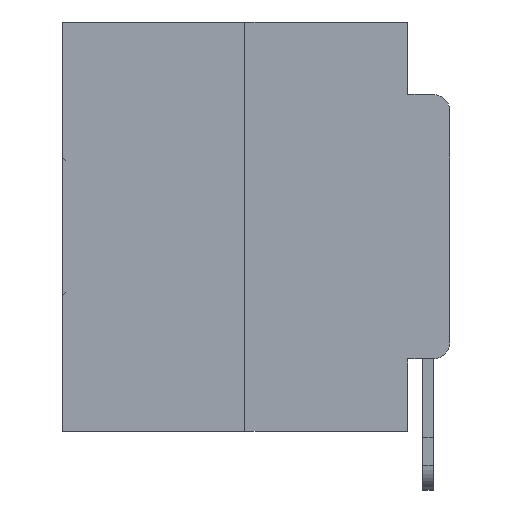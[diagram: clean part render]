
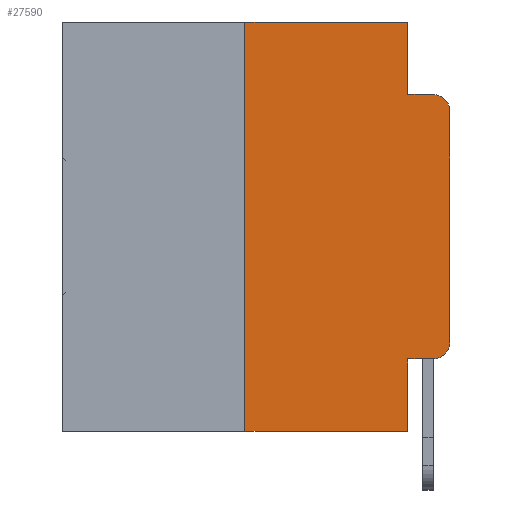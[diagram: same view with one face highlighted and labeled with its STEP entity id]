
A CAD part, left-side view. The second image highlights one B-rep face of the part: STEP entity #27590.
In plain terms, the highlighted planar face has unit normal (-1, 0, 0).
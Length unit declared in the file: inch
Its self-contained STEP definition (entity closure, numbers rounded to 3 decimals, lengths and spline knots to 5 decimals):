
#159 = DIRECTION ( 'NONE',  ( 0., -1., 0. ) ) ;
#421 = EDGE_CURVE ( 'NONE', #21652, #29234, #27852, .T. ) ;
#445 = ORIENTED_EDGE ( 'NONE', *, *, #11988, .T. ) ;
#767 = EDGE_CURVE ( 'NONE', #23382, #13753, #8471, .T. ) ;
#1017 = LINE ( 'NONE', #3094, #6237 ) ;
#1103 = CARTESIAN_POINT ( 'NONE',  ( 0., 0.051, -0.4115 ) ) ;
#1565 = ORIENTED_EDGE ( 'NONE', *, *, #421, .T. ) ;
#3057 = LINE ( 'NONE', #16010, #3883 ) ;
#3094 = CARTESIAN_POINT ( 'NONE',  ( 0., 0.25, 0. ) ) ;
#3330 = CARTESIAN_POINT ( 'NONE',  ( 0., 0.051, 0. ) ) ;
#3883 = VECTOR ( 'NONE', #29842, 39.37008 ) ;
#3971 = CIRCLE ( 'NONE', #16926, 0.02 ) ;
#3992 = ORIENTED_EDGE ( 'NONE', *, *, #29808, .F. ) ;
#4170 = AXIS2_PLACEMENT_3D ( 'NONE', #18735, #4355, #21090 ) ;
#4355 = DIRECTION ( 'NONE',  ( -1., 0., 0. ) ) ;
#5040 = VERTEX_POINT ( 'NONE', #10767 ) ;
#5738 = VERTEX_POINT ( 'NONE', #11638 ) ;
#6237 = VECTOR ( 'NONE', #15291, 39.37008 ) ;
#7415 = LINE ( 'NONE', #14215, #30066 ) ;
#7558 = CARTESIAN_POINT ( 'NONE',  ( 0., 0., 0. ) ) ;
#7598 = CARTESIAN_POINT ( 'NONE',  ( 0., 0.25, 0. ) ) ;
#7911 = PLANE ( 'NONE',  #27528 ) ;
#8407 = DIRECTION ( 'NONE',  ( 0., 0., -1. ) ) ;
#8471 = LINE ( 'NONE', #19296, #27109 ) ;
#8512 = EDGE_CURVE ( 'NONE', #14892, #15529, #7415, .T. ) ;
#9954 = ORIENTED_EDGE ( 'NONE', *, *, #8512, .T. ) ;
#10033 = VERTEX_POINT ( 'NONE', #21681 ) ;
#10429 = DIRECTION ( 'NONE',  ( 0., 0., -1. ) ) ;
#10767 = CARTESIAN_POINT ( 'NONE',  ( 0., 0.051, -0.0885 ) ) ;
#10844 = LINE ( 'NONE', #20130, #21762 ) ;
#11638 = CARTESIAN_POINT ( 'NONE',  ( 0., 0., -0.3915 ) ) ;
#11988 = EDGE_CURVE ( 'NONE', #5738, #10033, #22159, .T. ) ;
#12777 = EDGE_CURVE ( 'NONE', #13753, #5040, #10844, .T. ) ;
#13014 = CARTESIAN_POINT ( 'NONE',  ( 0., 0.02, -0.3915 ) ) ;
#13753 = VERTEX_POINT ( 'NONE', #20800 ) ;
#14215 = CARTESIAN_POINT ( 'NONE',  ( 0., 0.473, -0.5 ) ) ;
#14318 = CARTESIAN_POINT ( 'NONE',  ( 0., 0.051, -0.5 ) ) ;
#14400 = FACE_OUTER_BOUND ( 'NONE', #30806, .T. ) ;
#14892 = VERTEX_POINT ( 'NONE', #26892 ) ;
#15018 = CARTESIAN_POINT ( 'NONE',  ( 0., 0.473, 0. ) ) ;
#15291 = DIRECTION ( 'NONE',  ( 0., 0., 1. ) ) ;
#15359 = DIRECTION ( 'NONE',  ( 0., 0., -1. ) ) ;
#15529 = VERTEX_POINT ( 'NONE', #14318 ) ;
#15917 = CARTESIAN_POINT ( 'NONE',  ( 0., 0.02, -0.4115 ) ) ;
#16010 = CARTESIAN_POINT ( 'NONE',  ( 0., 0.051, -0.0885 ) ) ;
#16163 = ORIENTED_EDGE ( 'NONE', *, *, #767, .F. ) ;
#16926 = AXIS2_PLACEMENT_3D ( 'NONE', #13014, #29201, #15359 ) ;
#18274 = CARTESIAN_POINT ( 'NONE',  ( 0., 0.02, -0.0885 ) ) ;
#18735 = CARTESIAN_POINT ( 'NONE',  ( 0., 0.02, -0.1085 ) ) ;
#19296 = CARTESIAN_POINT ( 'NONE',  ( 0., 0.473, 0. ) ) ;
#19758 = EDGE_CURVE ( 'NONE', #10033, #30638, #20599, .T. ) ;
#20130 = CARTESIAN_POINT ( 'NONE',  ( 0., 0.051, 0. ) ) ;
#20512 = ORIENTED_EDGE ( 'NONE', *, *, #22132, .F. ) ;
#20599 = CIRCLE ( 'NONE', #4170, 0.02 ) ;
#20800 = CARTESIAN_POINT ( 'NONE',  ( 0., 0.051, 0. ) ) ;
#20803 = EDGE_CURVE ( 'NONE', #29234, #5738, #3971, .T. ) ;
#20974 = ORIENTED_EDGE ( 'NONE', *, *, #12777, .F. ) ;
#21006 = VECTOR ( 'NONE', #159, 39.37008 ) ;
#21090 = DIRECTION ( 'NONE',  ( 0., 0., -1. ) ) ;
#21322 = ORIENTED_EDGE ( 'NONE', *, *, #19758, .T. ) ;
#21652 = VERTEX_POINT ( 'NONE', #1103 ) ;
#21681 = CARTESIAN_POINT ( 'NONE',  ( 0., 0., -0.1085 ) ) ;
#21743 = EDGE_CURVE ( 'NONE', #5040, #30638, #3057, .T. ) ;
#21762 = VECTOR ( 'NONE', #8407, 39.37008 ) ;
#21850 = DIRECTION ( 'NONE',  ( 0., -1., 0. ) ) ;
#21956 = VECTOR ( 'NONE', #24805, 39.37008 ) ;
#22132 = EDGE_CURVE ( 'NONE', #14892, #23382, #1017, .T. ) ;
#22135 = ORIENTED_EDGE ( 'NONE', *, *, #21743, .F. ) ;
#22159 = LINE ( 'NONE', #7558, #27558 ) ;
#23382 = VERTEX_POINT ( 'NONE', #7598 ) ;
#24335 = DIRECTION ( 'NONE',  ( 1., 0., 0. ) ) ;
#24805 = DIRECTION ( 'NONE',  ( 0., 0., -1. ) ) ;
#26892 = CARTESIAN_POINT ( 'NONE',  ( 0., 0.25, -0.5 ) ) ;
#26983 = ORIENTED_EDGE ( 'NONE', *, *, #20803, .T. ) ;
#27109 = VECTOR ( 'NONE', #21850, 39.37008 ) ;
#27528 = AXIS2_PLACEMENT_3D ( 'NONE', #15018, #24335, #10429 ) ;
#27558 = VECTOR ( 'NONE', #30908, 39.37008 ) ;
#27590 = ADVANCED_FACE ( 'NONE', ( #14400 ), #7911, .F. ) ;
#27852 = LINE ( 'NONE', #30539, #21006 ) ;
#28075 = LINE ( 'NONE', #3330, #21956 ) ;
#29201 = DIRECTION ( 'NONE',  ( -1., 0., 0. ) ) ;
#29234 = VERTEX_POINT ( 'NONE', #15917 ) ;
#29808 = EDGE_CURVE ( 'NONE', #21652, #15529, #28075, .T. ) ;
#29842 = DIRECTION ( 'NONE',  ( 0., -1., 0. ) ) ;
#30066 = VECTOR ( 'NONE', #30373, 39.37008 ) ;
#30373 = DIRECTION ( 'NONE',  ( 0., -1., 0. ) ) ;
#30539 = CARTESIAN_POINT ( 'NONE',  ( 0., 0.051, -0.4115 ) ) ;
#30638 = VERTEX_POINT ( 'NONE', #18274 ) ;
#30806 = EDGE_LOOP ( 'NONE', ( #445, #21322, #22135, #20974, #16163, #20512, #9954, #3992, #1565, #26983 ) ) ;
#30908 = DIRECTION ( 'NONE',  ( 0., 0., 1. ) ) ;
